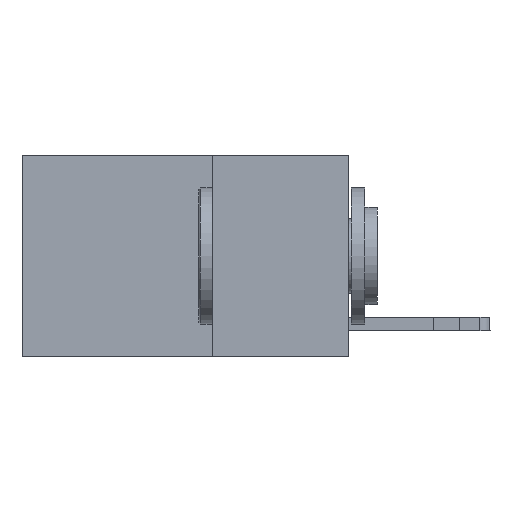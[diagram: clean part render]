
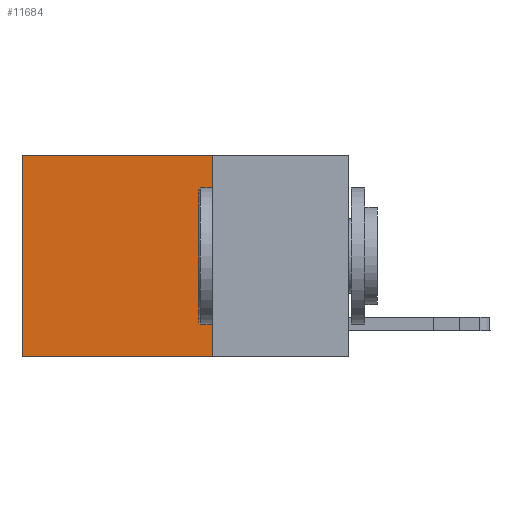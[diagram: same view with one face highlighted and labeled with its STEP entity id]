
A CAD part, left-side view. The second image highlights one B-rep face of the part: STEP entity #11684.
In plain terms, the highlighted planar face has unit normal (-1, 0, 0).
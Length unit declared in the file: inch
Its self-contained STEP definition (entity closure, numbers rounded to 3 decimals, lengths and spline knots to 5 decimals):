
#98 = FACE_OUTER_BOUND ( 'NONE', #12046, .T. ) ;
#478 = DIRECTION ( 'NONE',  ( 0., 0., -1. ) ) ;
#597 = EDGE_CURVE ( 'NONE', #2999, #8301, #12513, .T. ) ;
#1364 = ORIENTED_EDGE ( 'NONE', *, *, #7374, .T. ) ;
#1488 = EDGE_CURVE ( 'NONE', #8301, #18699, #12691, .T. ) ;
#1617 = CARTESIAN_POINT ( 'NONE',  ( 0.2625, 0.25, 0. ) ) ;
#1727 = DIRECTION ( 'NONE',  ( 0., 1., 0. ) ) ;
#1858 = DIRECTION ( 'NONE',  ( 1., 0., 0. ) ) ;
#2182 = DIRECTION ( 'NONE',  ( 0., 0., -1. ) ) ;
#2215 = ORIENTED_EDGE ( 'NONE', *, *, #1488, .F. ) ;
#2801 = CARTESIAN_POINT ( 'NONE',  ( 0.2625, 0.25, -0.37 ) ) ;
#2999 = VERTEX_POINT ( 'NONE', #4876 ) ;
#3896 = VECTOR ( 'NONE', #1727, 39.37008 ) ;
#4033 = VECTOR ( 'NONE', #478, 39.37008 ) ;
#4736 = CARTESIAN_POINT ( 'NONE',  ( 0.2625, 0.6, 0. ) ) ;
#4876 = CARTESIAN_POINT ( 'NONE',  ( 0.2625, 0.25, 0. ) ) ;
#5234 = AXIS2_PLACEMENT_3D ( 'NONE', #8639, #1858, #2182 ) ;
#6317 = DIRECTION ( 'NONE',  ( 0., 1., 0. ) ) ;
#7374 = EDGE_CURVE ( 'NONE', #11145, #18699, #17295, .T. ) ;
#8301 = VERTEX_POINT ( 'NONE', #18892 ) ;
#8308 = LINE ( 'NONE', #1617, #3896 ) ;
#8639 = CARTESIAN_POINT ( 'NONE',  ( 0.2625, 0.25, 0. ) ) ;
#9340 = DIRECTION ( 'NONE',  ( 0., 0., -1. ) ) ;
#9491 = ORIENTED_EDGE ( 'NONE', *, *, #13003, .T. ) ;
#11145 = VERTEX_POINT ( 'NONE', #4736 ) ;
#11684 = ADVANCED_FACE ( 'NONE', ( #98 ), #18893, .F. ) ;
#12007 = CARTESIAN_POINT ( 'NONE',  ( 0.2625, 0.6, 0. ) ) ;
#12046 = EDGE_LOOP ( 'NONE', ( #1364, #2215, #14251, #9491 ) ) ;
#12239 = VECTOR ( 'NONE', #6317, 39.37008 ) ;
#12513 = LINE ( 'NONE', #19243, #19028 ) ;
#12691 = LINE ( 'NONE', #2801, #12239 ) ;
#13003 = EDGE_CURVE ( 'NONE', #2999, #11145, #8308, .T. ) ;
#14251 = ORIENTED_EDGE ( 'NONE', *, *, #597, .F. ) ;
#14817 = CARTESIAN_POINT ( 'NONE',  ( 0.2625, 0.6, -0.37 ) ) ;
#17295 = LINE ( 'NONE', #12007, #4033 ) ;
#18699 = VERTEX_POINT ( 'NONE', #14817 ) ;
#18892 = CARTESIAN_POINT ( 'NONE',  ( 0.2625, 0.25, -0.37 ) ) ;
#18893 = PLANE ( 'NONE',  #5234 ) ;
#19028 = VECTOR ( 'NONE', #9340, 39.37008 ) ;
#19243 = CARTESIAN_POINT ( 'NONE',  ( 0.2625, 0.25, 0. ) ) ;
